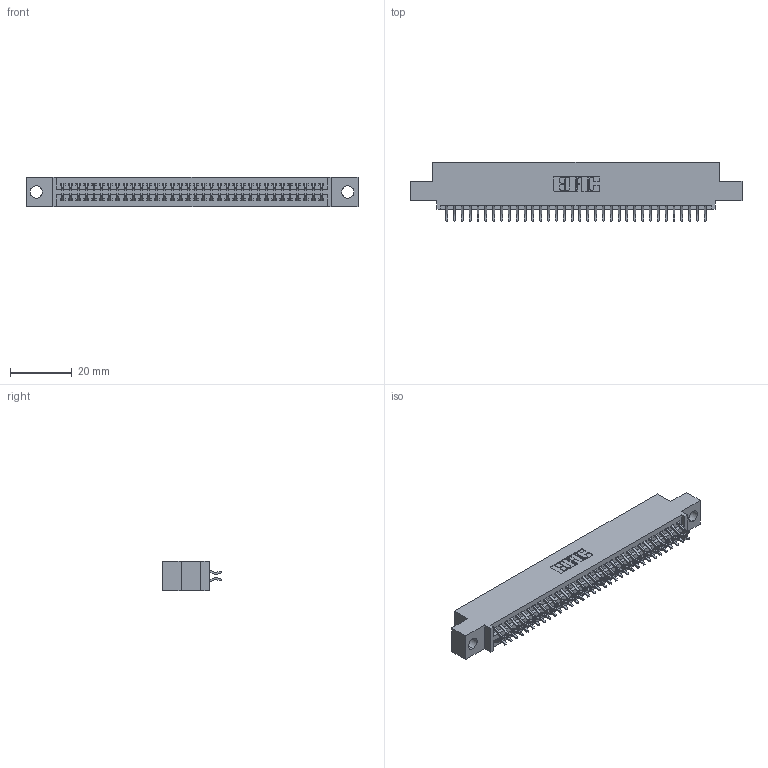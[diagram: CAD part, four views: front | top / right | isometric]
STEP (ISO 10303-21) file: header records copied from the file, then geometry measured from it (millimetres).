
FILE_DESCRIPTION (( 'STEP AP203' ), '1' );
FILE_NAME ('395-068-556-504.STEP', '2018-11-25T19:00:04', ( '' ), ( '' ), 'SwSTEP 2.0', 'SolidWorks 2016', '' );
FILE_SCHEMA (( 'CONFIG_CONTROL_DESIGN' ));
Length unit declared in the file: inch
Products named in the file (3): 345 Part_0.110 Offset - 0.156 Dia-TH; 345-292-001_556 Tail; 395-068-556-504
Assembly tree (69 placements, depth 2):
  395-068-556-504
    345 Part_0.110 Offset - 0.156 Dia-TH
    345-292-001_556 Tail  x68
Bounding box: 107.57 x 19.24 x 9.4 mm (x, y, z)
Volume: 10211.2 mm3; surface area: 14787.4 mm2
Topology: 69 solids, 69 shells, 3938 faces, 11709 edges, 7714 vertices
Faces by surface type: plane 2600, cylinder 1338
Entity records: 28109 total; most frequent: CARTESIAN_POINT 4736, ORIENTED_EDGE 4658, DIRECTION 4173, EDGE_CURVE 2329, VECTOR 2053, LINE 2053, VERTEX_POINT 1550, AXIS2_PLACEMENT_3D 1060
